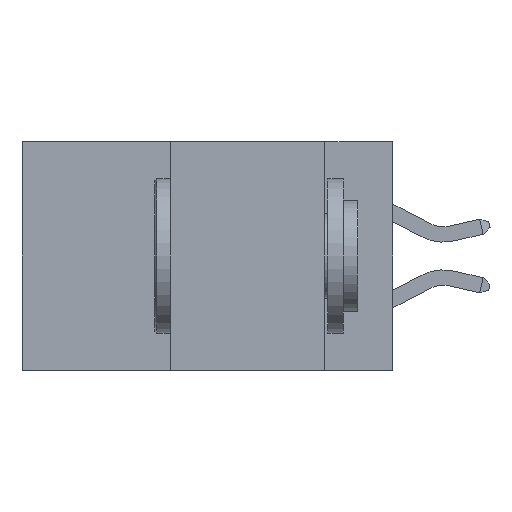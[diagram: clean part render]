
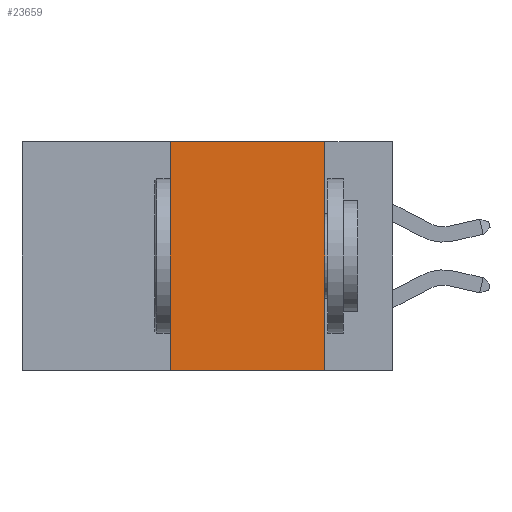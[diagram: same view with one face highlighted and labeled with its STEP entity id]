
A CAD part, left-side view. The second image highlights one B-rep face of the part: STEP entity #23659.
In plain terms, the highlighted planar face has unit normal (-1, 0, 0).
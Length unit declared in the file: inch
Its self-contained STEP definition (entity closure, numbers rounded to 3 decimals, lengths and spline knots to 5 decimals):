
#1179 = EDGE_CURVE ( 'NONE', #24055, #13958, #20688, .T. ) ;
#1612 = CARTESIAN_POINT ( 'NONE',  ( 0., 0.11, 0. ) ) ;
#3083 = LINE ( 'NONE', #19123, #7889 ) ;
#3117 = ORIENTED_EDGE ( 'NONE', *, *, #9704, .F. ) ;
#3932 = EDGE_CURVE ( 'NONE', #18948, #16513, #3083, .T. ) ;
#3992 = CARTESIAN_POINT ( 'NONE',  ( 0., 0.36, 0. ) ) ;
#4372 = AXIS2_PLACEMENT_3D ( 'NONE', #15637, #17420, #5924 ) ;
#4767 = VECTOR ( 'NONE', #8908, 39.37008 ) ;
#5924 = DIRECTION ( 'NONE',  ( 0., 0., -1. ) ) ;
#6192 = VECTOR ( 'NONE', #18928, 39.37008 ) ;
#7446 = FACE_OUTER_BOUND ( 'NONE', #9588, .T. ) ;
#7889 = VECTOR ( 'NONE', #22880, 39.37008 ) ;
#8908 = DIRECTION ( 'NONE',  ( 0., -1., 0. ) ) ;
#9224 = ORIENTED_EDGE ( 'NONE', *, *, #3932, .F. ) ;
#9588 = EDGE_LOOP ( 'NONE', ( #16837, #3117, #9224, #21973 ) ) ;
#9704 = EDGE_CURVE ( 'NONE', #16513, #24055, #16170, .T. ) ;
#9793 = PLANE ( 'NONE',  #4372 ) ;
#11721 = LINE ( 'NONE', #12686, #18996 ) ;
#12686 = CARTESIAN_POINT ( 'NONE',  ( 0., 0.6, -0.37 ) ) ;
#13958 = VERTEX_POINT ( 'NONE', #20467 ) ;
#14516 = DIRECTION ( 'NONE',  ( 0., -1., 0. ) ) ;
#15637 = CARTESIAN_POINT ( 'NONE',  ( 0., 0.6, 0. ) ) ;
#16170 = LINE ( 'NONE', #18665, #4767 ) ;
#16513 = VERTEX_POINT ( 'NONE', #3992 ) ;
#16837 = ORIENTED_EDGE ( 'NONE', *, *, #1179, .F. ) ;
#17420 = DIRECTION ( 'NONE',  ( 1., 0., 0. ) ) ;
#18665 = CARTESIAN_POINT ( 'NONE',  ( 0., 0.6, 0. ) ) ;
#18790 = CARTESIAN_POINT ( 'NONE',  ( 0., 0.11, 0. ) ) ;
#18928 = DIRECTION ( 'NONE',  ( 0., 0., -1. ) ) ;
#18948 = VERTEX_POINT ( 'NONE', #24110 ) ;
#18970 = EDGE_CURVE ( 'NONE', #18948, #13958, #11721, .T. ) ;
#18996 = VECTOR ( 'NONE', #14516, 39.37008 ) ;
#19123 = CARTESIAN_POINT ( 'NONE',  ( 0., 0.36, 0. ) ) ;
#20467 = CARTESIAN_POINT ( 'NONE',  ( 0., 0.11, -0.37 ) ) ;
#20688 = LINE ( 'NONE', #1612, #6192 ) ;
#21973 = ORIENTED_EDGE ( 'NONE', *, *, #18970, .T. ) ;
#22880 = DIRECTION ( 'NONE',  ( 0., 0., 1. ) ) ;
#23659 = ADVANCED_FACE ( 'NONE', ( #7446 ), #9793, .F. ) ;
#24055 = VERTEX_POINT ( 'NONE', #18790 ) ;
#24110 = CARTESIAN_POINT ( 'NONE',  ( 0., 0.36, -0.37 ) ) ;
